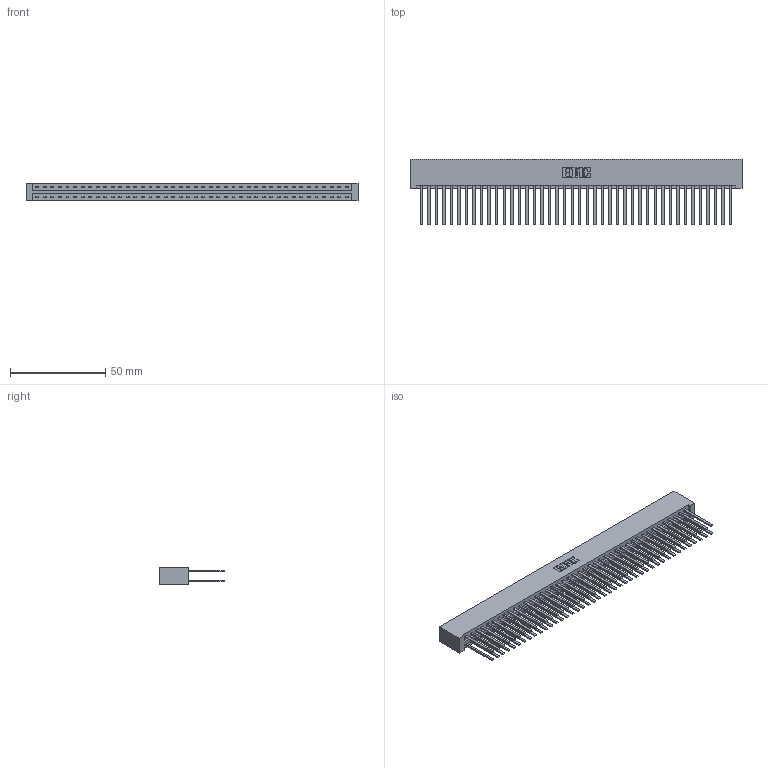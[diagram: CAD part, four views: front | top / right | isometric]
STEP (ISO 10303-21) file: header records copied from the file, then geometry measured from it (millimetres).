
FILE_DESCRIPTION (( 'STEP AP203' ), '1' );
FILE_NAME ('337-084-544-201.STEP', '2019-10-10T14:08:39', ( '' ), ( '' ), 'SwSTEP 2.0', 'SolidWorks 2016', '' );
FILE_SCHEMA (( 'CONFIG_CONTROL_DESIGN' ));
Length unit declared in the file: inch
Products named in the file (3): 345-292-001_345-293-144; 337-084-544-201; 337 Part_No Mounting Lugs
Assembly tree (85 placements, depth 2):
  337-084-544-201
    337 Part_No Mounting Lugs
    345-292-001_345-293-144  x84
Bounding box: 174.29 x 34.3 x 9.4 mm (x, y, z)
Volume: 20306.8 mm3; surface area: 26859.7 mm2
Topology: 85 solids, 85 shells, 4138 faces, 12299 edges, 8086 vertices
Faces by surface type: plane 2922, cylinder 1216
Entity records: 32103 total; most frequent: CARTESIAN_POINT 5406, ORIENTED_EDGE 5342, DIRECTION 4587, EDGE_CURVE 2671, LINE 2555, VECTOR 2555, VERTEX_POINT 1778, AXIS2_PLACEMENT_3D 1016
